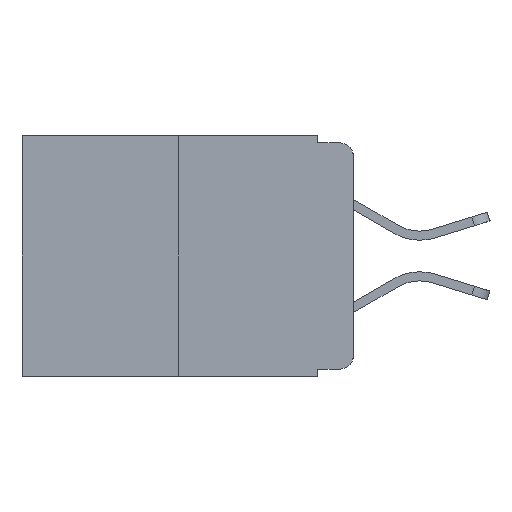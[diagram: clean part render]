
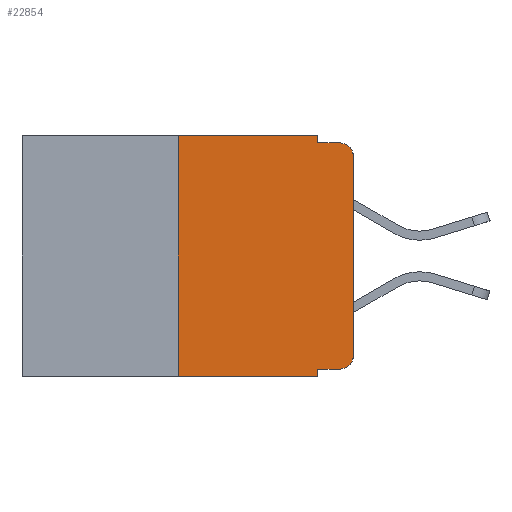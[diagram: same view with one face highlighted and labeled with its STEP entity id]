
A CAD part, left-side view. The second image highlights one B-rep face of the part: STEP entity #22854.
In plain terms, the highlighted planar face has unit normal (-1, 0, 0).
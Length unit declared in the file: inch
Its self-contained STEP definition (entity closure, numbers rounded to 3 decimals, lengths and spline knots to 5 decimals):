
#114 = VERTEX_POINT ( 'NONE', #8776 ) ;
#993 = CARTESIAN_POINT ( 'NONE',  ( 0., 0.25, -0.343 ) ) ;
#1153 = VECTOR ( 'NONE', #4797, 39.37008 ) ;
#1374 = CARTESIAN_POINT ( 'NONE',  ( 0., 0.051, -0.01 ) ) ;
#1442 = DIRECTION ( 'NONE',  ( 1., 0., 0. ) ) ;
#1578 = CIRCLE ( 'NONE', #7462, 0.02 ) ;
#1750 = LINE ( 'NONE', #2900, #1153 ) ;
#1971 = EDGE_CURVE ( 'NONE', #3281, #5273, #22069, .T. ) ;
#2463 = ORIENTED_EDGE ( 'NONE', *, *, #11676, .F. ) ;
#2483 = ORIENTED_EDGE ( 'NONE', *, *, #7172, .T. ) ;
#2488 = DIRECTION ( 'NONE',  ( 0., 0., 1. ) ) ;
#2900 = CARTESIAN_POINT ( 'NONE',  ( 0., 0.473, -0.343 ) ) ;
#3281 = VERTEX_POINT ( 'NONE', #993 ) ;
#3722 = EDGE_CURVE ( 'NONE', #23732, #4732, #13948, .T. ) ;
#4207 = CARTESIAN_POINT ( 'NONE',  ( 0., 0.02, -0.03 ) ) ;
#4277 = LINE ( 'NONE', #15344, #4862 ) ;
#4514 = EDGE_CURVE ( 'NONE', #5904, #19916, #14515, .T. ) ;
#4732 = VERTEX_POINT ( 'NONE', #21338 ) ;
#4797 = DIRECTION ( 'NONE',  ( 0., -1., 0. ) ) ;
#4862 = VECTOR ( 'NONE', #7398, 39.37008 ) ;
#5273 = VERTEX_POINT ( 'NONE', #9358 ) ;
#5623 = VECTOR ( 'NONE', #24326, 39.37008 ) ;
#5770 = ORIENTED_EDGE ( 'NONE', *, *, #10319, .T. ) ;
#5904 = VERTEX_POINT ( 'NONE', #24869 ) ;
#5933 = EDGE_CURVE ( 'NONE', #5273, #21860, #4277, .T. ) ;
#6019 = VERTEX_POINT ( 'NONE', #11661 ) ;
#6447 = VECTOR ( 'NONE', #15104, 39.37008 ) ;
#6759 = CARTESIAN_POINT ( 'NONE',  ( 0., 0.051, -0.01 ) ) ;
#6796 = LINE ( 'NONE', #9241, #21796 ) ;
#7172 = EDGE_CURVE ( 'NONE', #19916, #6019, #1578, .T. ) ;
#7398 = DIRECTION ( 'NONE',  ( 0., -1., 0. ) ) ;
#7462 = AXIS2_PLACEMENT_3D ( 'NONE', #20850, #9132, #22790 ) ;
#7728 = CARTESIAN_POINT ( 'NONE',  ( 0., 0.473, 0. ) ) ;
#7936 = ORIENTED_EDGE ( 'NONE', *, *, #3722, .T. ) ;
#8080 = FACE_OUTER_BOUND ( 'NONE', #17645, .T. ) ;
#8615 = VECTOR ( 'NONE', #14957, 39.37008 ) ;
#8776 = CARTESIAN_POINT ( 'NONE',  ( 0., 0.051, -0.343 ) ) ;
#8914 = VECTOR ( 'NONE', #21884, 39.37008 ) ;
#8988 = LINE ( 'NONE', #23865, #18238 ) ;
#9132 = DIRECTION ( 'NONE',  ( -1., 0., 0. ) ) ;
#9241 = CARTESIAN_POINT ( 'NONE',  ( 0., 0.051, 0. ) ) ;
#9358 = CARTESIAN_POINT ( 'NONE',  ( 0., 0.25, 0. ) ) ;
#9602 = EDGE_CURVE ( 'NONE', #3281, #114, #1750, .T. ) ;
#10319 = EDGE_CURVE ( 'NONE', #6019, #23732, #8988, .T. ) ;
#11661 = CARTESIAN_POINT ( 'NONE',  ( 0., 0., -0.313 ) ) ;
#11676 = EDGE_CURVE ( 'NONE', #21860, #24479, #14218, .T. ) ;
#11741 = PLANE ( 'NONE',  #15269 ) ;
#12007 = ORIENTED_EDGE ( 'NONE', *, *, #9602, .T. ) ;
#12841 = CARTESIAN_POINT ( 'NONE',  ( 0., 0., -0.03 ) ) ;
#12894 = AXIS2_PLACEMENT_3D ( 'NONE', #4207, #13783, #16542 ) ;
#13003 = CARTESIAN_POINT ( 'NONE',  ( 0., 0.051, -0.333 ) ) ;
#13718 = DIRECTION ( 'NONE',  ( 0., 0., -1. ) ) ;
#13783 = DIRECTION ( 'NONE',  ( -1., 0., 0. ) ) ;
#13948 = CIRCLE ( 'NONE', #12894, 0.02 ) ;
#14218 = LINE ( 'NONE', #23734, #8914 ) ;
#14303 = EDGE_CURVE ( 'NONE', #24479, #4732, #21256, .T. ) ;
#14515 = LINE ( 'NONE', #13003, #8615 ) ;
#14582 = CARTESIAN_POINT ( 'NONE',  ( 0., 0.25, 0. ) ) ;
#14957 = DIRECTION ( 'NONE',  ( 0., -1., 0. ) ) ;
#15104 = DIRECTION ( 'NONE',  ( 0., 0., 1. ) ) ;
#15269 = AXIS2_PLACEMENT_3D ( 'NONE', #7728, #1442, #13718 ) ;
#15344 = CARTESIAN_POINT ( 'NONE',  ( 0., 0.473, 0. ) ) ;
#15360 = ORIENTED_EDGE ( 'NONE', *, *, #5933, .F. ) ;
#16299 = ORIENTED_EDGE ( 'NONE', *, *, #23356, .F. ) ;
#16542 = DIRECTION ( 'NONE',  ( 0., 0., -1. ) ) ;
#17525 = ORIENTED_EDGE ( 'NONE', *, *, #4514, .T. ) ;
#17645 = EDGE_LOOP ( 'NONE', ( #5770, #7936, #24084, #2463, #15360, #21700, #12007, #16299, #17525, #2483 ) ) ;
#18238 = VECTOR ( 'NONE', #2488, 39.37008 ) ;
#19916 = VERTEX_POINT ( 'NONE', #24596 ) ;
#20850 = CARTESIAN_POINT ( 'NONE',  ( 0., 0.02, -0.313 ) ) ;
#20951 = DIRECTION ( 'NONE',  ( 0., 0., -1. ) ) ;
#21256 = LINE ( 'NONE', #6759, #5623 ) ;
#21338 = CARTESIAN_POINT ( 'NONE',  ( 0., 0.02, -0.01 ) ) ;
#21700 = ORIENTED_EDGE ( 'NONE', *, *, #1971, .F. ) ;
#21796 = VECTOR ( 'NONE', #20951, 39.37008 ) ;
#21860 = VERTEX_POINT ( 'NONE', #24752 ) ;
#21884 = DIRECTION ( 'NONE',  ( 0., 0., -1. ) ) ;
#22069 = LINE ( 'NONE', #14582, #6447 ) ;
#22790 = DIRECTION ( 'NONE',  ( 0., 0., -1. ) ) ;
#22854 = ADVANCED_FACE ( 'NONE', ( #8080 ), #11741, .F. ) ;
#23356 = EDGE_CURVE ( 'NONE', #5904, #114, #6796, .T. ) ;
#23732 = VERTEX_POINT ( 'NONE', #12841 ) ;
#23734 = CARTESIAN_POINT ( 'NONE',  ( 0., 0.051, 0. ) ) ;
#23865 = CARTESIAN_POINT ( 'NONE',  ( 0., 0., 0. ) ) ;
#24084 = ORIENTED_EDGE ( 'NONE', *, *, #14303, .F. ) ;
#24326 = DIRECTION ( 'NONE',  ( 0., -1., 0. ) ) ;
#24479 = VERTEX_POINT ( 'NONE', #1374 ) ;
#24596 = CARTESIAN_POINT ( 'NONE',  ( 0., 0.02, -0.333 ) ) ;
#24752 = CARTESIAN_POINT ( 'NONE',  ( 0., 0.051, 0. ) ) ;
#24869 = CARTESIAN_POINT ( 'NONE',  ( 0., 0.051, -0.333 ) ) ;
